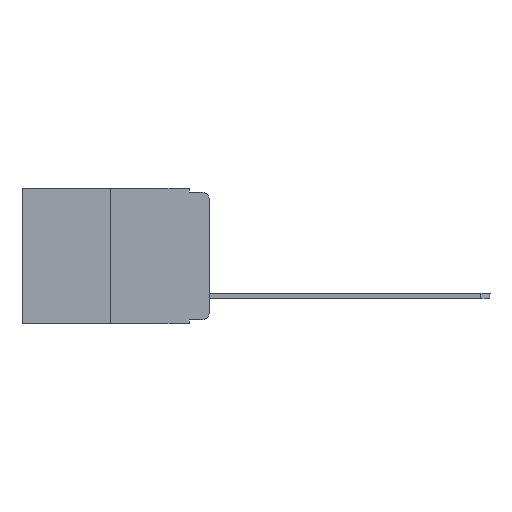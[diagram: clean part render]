
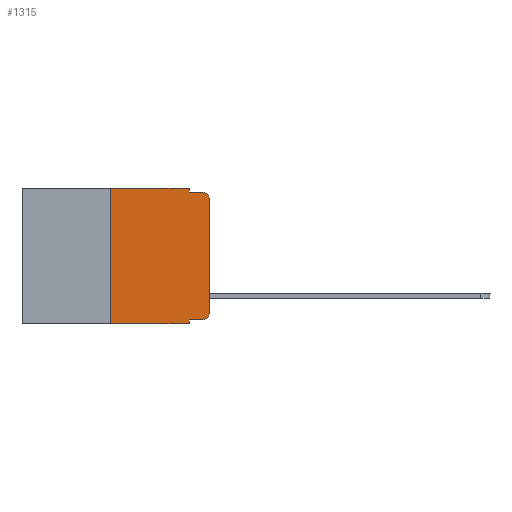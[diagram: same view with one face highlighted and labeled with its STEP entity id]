
A CAD part, left-side view. The second image highlights one B-rep face of the part: STEP entity #1315.
In plain terms, the highlighted planar face has unit normal (-1, 0, 0).
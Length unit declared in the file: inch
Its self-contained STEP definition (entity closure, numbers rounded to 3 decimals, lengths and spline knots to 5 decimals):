
#116 = PLANE ( 'NONE',  #5310 ) ;
#209 = LINE ( 'NONE', #7983, #1612 ) ;
#500 = CARTESIAN_POINT ( 'NONE',  ( 0., 0.051, 0. ) ) ;
#716 = EDGE_LOOP ( 'NONE', ( #2681, #8772, #4163, #758, #2357, #7244, #3638, #4492, #4983, #6620 ) ) ;
#758 = ORIENTED_EDGE ( 'NONE', *, *, #4284, .F. ) ;
#857 = CARTESIAN_POINT ( 'NONE',  ( 0., 0.051, -0.333 ) ) ;
#893 = CIRCLE ( 'NONE', #8588, 0.02 ) ;
#1315 = ADVANCED_FACE ( 'NONE', ( #6749 ), #116, .F. ) ;
#1486 = LINE ( 'NONE', #4434, #3362 ) ;
#1507 = CARTESIAN_POINT ( 'NONE',  ( 0., 0.02, -0.333 ) ) ;
#1612 = VECTOR ( 'NONE', #2084, 39.37008 ) ;
#1615 = DIRECTION ( 'NONE',  ( 1., 0., 0. ) ) ;
#2082 = CARTESIAN_POINT ( 'NONE',  ( 0., 0.473, -0.343 ) ) ;
#2084 = DIRECTION ( 'NONE',  ( 0., -1., 0. ) ) ;
#2315 = EDGE_CURVE ( 'NONE', #5889, #4862, #1486, .T. ) ;
#2357 = ORIENTED_EDGE ( 'NONE', *, *, #8804, .F. ) ;
#2662 = DIRECTION ( 'NONE',  ( 0., -1., 0. ) ) ;
#2681 = ORIENTED_EDGE ( 'NONE', *, *, #2945, .T. ) ;
#2751 = LINE ( 'NONE', #4169, #5513 ) ;
#2781 = VERTEX_POINT ( 'NONE', #4792 ) ;
#2943 = EDGE_CURVE ( 'NONE', #4159, #2781, #7981, .T. ) ;
#2945 = EDGE_CURVE ( 'NONE', #6643, #8765, #2751, .T. ) ;
#2955 = VERTEX_POINT ( 'NONE', #500 ) ;
#2984 = CARTESIAN_POINT ( 'NONE',  ( 0., 0., -0.313 ) ) ;
#3052 = CIRCLE ( 'NONE', #8916, 0.02 ) ;
#3220 = DIRECTION ( 'NONE',  ( 0., -1., 0. ) ) ;
#3362 = VECTOR ( 'NONE', #3220, 39.37008 ) ;
#3395 = DIRECTION ( 'NONE',  ( -1., 0., 0. ) ) ;
#3431 = DIRECTION ( 'NONE',  ( 0., 0., -1. ) ) ;
#3532 = CARTESIAN_POINT ( 'NONE',  ( 0., 0.051, 0. ) ) ;
#3609 = VECTOR ( 'NONE', #7840, 39.37008 ) ;
#3638 = ORIENTED_EDGE ( 'NONE', *, *, #2943, .T. ) ;
#3647 = EDGE_CURVE ( 'NONE', #4159, #3730, #8880, .T. ) ;
#3730 = VERTEX_POINT ( 'NONE', #6781 ) ;
#4159 = VERTEX_POINT ( 'NONE', #6979 ) ;
#4163 = ORIENTED_EDGE ( 'NONE', *, *, #4225, .F. ) ;
#4169 = CARTESIAN_POINT ( 'NONE',  ( 0., 0., 0. ) ) ;
#4225 = EDGE_CURVE ( 'NONE', #5991, #9440, #209, .T. ) ;
#4278 = VECTOR ( 'NONE', #2662, 39.37008 ) ;
#4284 = EDGE_CURVE ( 'NONE', #2955, #5991, #5089, .T. ) ;
#4434 = CARTESIAN_POINT ( 'NONE',  ( 0., 0.051, -0.333 ) ) ;
#4469 = CARTESIAN_POINT ( 'NONE',  ( 0., 0.473, 0. ) ) ;
#4492 = ORIENTED_EDGE ( 'NONE', *, *, #6500, .F. ) ;
#4510 = LINE ( 'NONE', #4469, #6288 ) ;
#4731 = VECTOR ( 'NONE', #8175, 39.37008 ) ;
#4792 = CARTESIAN_POINT ( 'NONE',  ( 0., 0.051, -0.343 ) ) ;
#4862 = VERTEX_POINT ( 'NONE', #1507 ) ;
#4983 = ORIENTED_EDGE ( 'NONE', *, *, #2315, .T. ) ;
#5089 = LINE ( 'NONE', #3532, #3609 ) ;
#5141 = DIRECTION ( 'NONE',  ( 0., 0., -1. ) ) ;
#5310 = AXIS2_PLACEMENT_3D ( 'NONE', #5816, #1615, #5141 ) ;
#5319 = DIRECTION ( 'NONE',  ( 0., 0., -1. ) ) ;
#5513 = VECTOR ( 'NONE', #7115, 39.37008 ) ;
#5816 = CARTESIAN_POINT ( 'NONE',  ( 0., 0.473, 0. ) ) ;
#5889 = VERTEX_POINT ( 'NONE', #857 ) ;
#5991 = VERTEX_POINT ( 'NONE', #6892 ) ;
#6044 = DIRECTION ( 'NONE',  ( -1., 0., 0. ) ) ;
#6237 = CARTESIAN_POINT ( 'NONE',  ( 0., 0.051, 0. ) ) ;
#6288 = VECTOR ( 'NONE', #8137, 39.37008 ) ;
#6401 = CARTESIAN_POINT ( 'NONE',  ( 0., 0.02, -0.03 ) ) ;
#6500 = EDGE_CURVE ( 'NONE', #5889, #2781, #8641, .T. ) ;
#6620 = ORIENTED_EDGE ( 'NONE', *, *, #8080, .T. ) ;
#6643 = VERTEX_POINT ( 'NONE', #2984 ) ;
#6747 = CARTESIAN_POINT ( 'NONE',  ( 0., 0., -0.03 ) ) ;
#6749 = FACE_OUTER_BOUND ( 'NONE', #716, .T. ) ;
#6759 = VECTOR ( 'NONE', #3431, 39.37008 ) ;
#6781 = CARTESIAN_POINT ( 'NONE',  ( 0., 0.25, 0. ) ) ;
#6892 = CARTESIAN_POINT ( 'NONE',  ( 0., 0.051, -0.01 ) ) ;
#6979 = CARTESIAN_POINT ( 'NONE',  ( 0., 0.25, -0.343 ) ) ;
#7115 = DIRECTION ( 'NONE',  ( 0., 0., 1. ) ) ;
#7244 = ORIENTED_EDGE ( 'NONE', *, *, #3647, .F. ) ;
#7331 = CARTESIAN_POINT ( 'NONE',  ( 0., 0.02, -0.01 ) ) ;
#7436 = EDGE_CURVE ( 'NONE', #8765, #9440, #3052, .T. ) ;
#7581 = CARTESIAN_POINT ( 'NONE',  ( 0., 0.02, -0.313 ) ) ;
#7840 = DIRECTION ( 'NONE',  ( 0., 0., -1. ) ) ;
#7981 = LINE ( 'NONE', #2082, #4278 ) ;
#7983 = CARTESIAN_POINT ( 'NONE',  ( 0., 0.051, -0.01 ) ) ;
#8080 = EDGE_CURVE ( 'NONE', #4862, #6643, #893, .T. ) ;
#8137 = DIRECTION ( 'NONE',  ( 0., -1., 0. ) ) ;
#8175 = DIRECTION ( 'NONE',  ( 0., 0., 1. ) ) ;
#8588 = AXIS2_PLACEMENT_3D ( 'NONE', #7581, #6044, #5319 ) ;
#8641 = LINE ( 'NONE', #6237, #6759 ) ;
#8765 = VERTEX_POINT ( 'NONE', #6747 ) ;
#8772 = ORIENTED_EDGE ( 'NONE', *, *, #7436, .T. ) ;
#8789 = CARTESIAN_POINT ( 'NONE',  ( 0., 0.25, 0. ) ) ;
#8804 = EDGE_CURVE ( 'NONE', #3730, #2955, #4510, .T. ) ;
#8880 = LINE ( 'NONE', #8789, #4731 ) ;
#8916 = AXIS2_PLACEMENT_3D ( 'NONE', #6401, #3395, #9434 ) ;
#9434 = DIRECTION ( 'NONE',  ( 0., 0., -1. ) ) ;
#9440 = VERTEX_POINT ( 'NONE', #7331 ) ;
